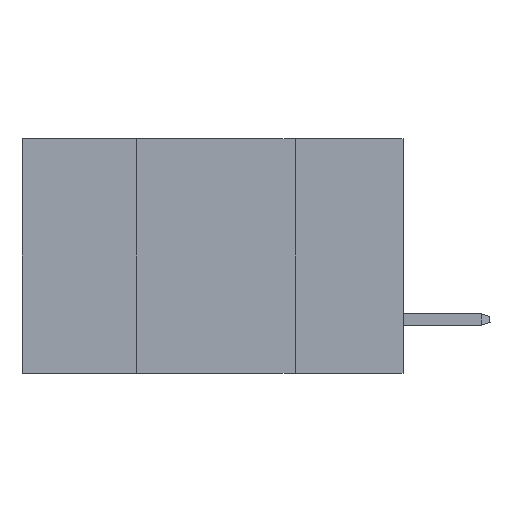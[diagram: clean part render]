
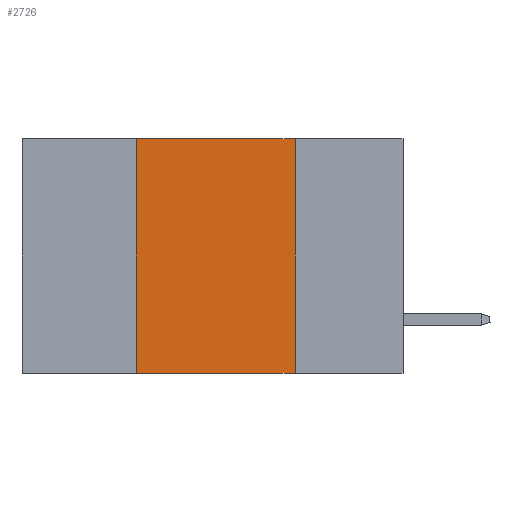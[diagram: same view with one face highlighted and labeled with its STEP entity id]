
A CAD part, left-side view. The second image highlights one B-rep face of the part: STEP entity #2726.
In plain terms, the highlighted planar face has unit normal (-1, 0, 0).
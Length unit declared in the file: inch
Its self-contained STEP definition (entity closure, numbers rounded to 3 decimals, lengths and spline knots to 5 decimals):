
#226 = EDGE_CURVE ( 'NONE', #13927, #16202, #13857, .T. ) ;
#305 = ORIENTED_EDGE ( 'NONE', *, *, #226, .F. ) ;
#566 = CARTESIAN_POINT ( 'NONE',  ( 0., 0.17, 0. ) ) ;
#1072 = DIRECTION ( 'NONE',  ( 0., 0., -1. ) ) ;
#1636 = LINE ( 'NONE', #4670, #15928 ) ;
#2726 = ADVANCED_FACE ( 'NONE', ( #11357 ), #4128, .F. ) ;
#3113 = EDGE_CURVE ( 'NONE', #11606, #16202, #15588, .T. ) ;
#3751 = CARTESIAN_POINT ( 'NONE',  ( 0., 0.42, 0. ) ) ;
#3967 = VECTOR ( 'NONE', #11288, 39.37008 ) ;
#4128 = PLANE ( 'NONE',  #17933 ) ;
#4250 = LINE ( 'NONE', #6941, #5107 ) ;
#4453 = CARTESIAN_POINT ( 'NONE',  ( 0., 0.17, -0.37 ) ) ;
#4670 = CARTESIAN_POINT ( 'NONE',  ( 0., 0.6, 0. ) ) ;
#5107 = VECTOR ( 'NONE', #5553, 39.37008 ) ;
#5553 = DIRECTION ( 'NONE',  ( 0., 0., 1. ) ) ;
#6872 = CARTESIAN_POINT ( 'NONE',  ( 0., 0.17, 0. ) ) ;
#6918 = CARTESIAN_POINT ( 'NONE',  ( 0., 0.6, 0. ) ) ;
#6941 = CARTESIAN_POINT ( 'NONE',  ( 0., 0.42, 0. ) ) ;
#7554 = VERTEX_POINT ( 'NONE', #3751 ) ;
#9192 = ORIENTED_EDGE ( 'NONE', *, *, #15597, .F. ) ;
#9497 = DIRECTION ( 'NONE',  ( 0., 0., -1. ) ) ;
#11288 = DIRECTION ( 'NONE',  ( 0., -1., 0. ) ) ;
#11357 = FACE_OUTER_BOUND ( 'NONE', #13627, .T. ) ;
#11382 = CARTESIAN_POINT ( 'NONE',  ( 0., 0.6, -0.37 ) ) ;
#11411 = DIRECTION ( 'NONE',  ( 0., -1., 0. ) ) ;
#11606 = VERTEX_POINT ( 'NONE', #11705 ) ;
#11705 = CARTESIAN_POINT ( 'NONE',  ( 0., 0.42, -0.37 ) ) ;
#13627 = EDGE_LOOP ( 'NONE', ( #305, #9192, #16306, #15169 ) ) ;
#13857 = LINE ( 'NONE', #6872, #15825 ) ;
#13927 = VERTEX_POINT ( 'NONE', #566 ) ;
#15169 = ORIENTED_EDGE ( 'NONE', *, *, #3113, .T. ) ;
#15354 = DIRECTION ( 'NONE',  ( 1., 0., 0. ) ) ;
#15588 = LINE ( 'NONE', #11382, #3967 ) ;
#15597 = EDGE_CURVE ( 'NONE', #7554, #13927, #1636, .T. ) ;
#15825 = VECTOR ( 'NONE', #1072, 39.37008 ) ;
#15928 = VECTOR ( 'NONE', #11411, 39.37008 ) ;
#16202 = VERTEX_POINT ( 'NONE', #4453 ) ;
#16306 = ORIENTED_EDGE ( 'NONE', *, *, #17814, .F. ) ;
#17814 = EDGE_CURVE ( 'NONE', #11606, #7554, #4250, .T. ) ;
#17933 = AXIS2_PLACEMENT_3D ( 'NONE', #6918, #15354, #9497 ) ;
